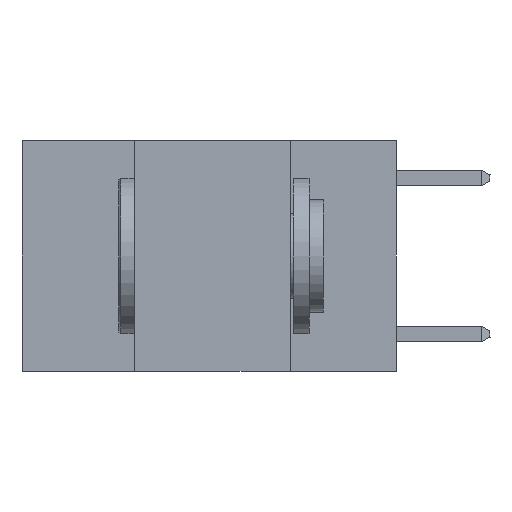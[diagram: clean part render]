
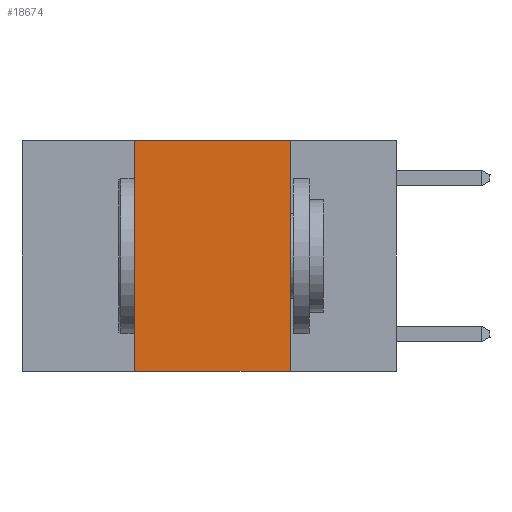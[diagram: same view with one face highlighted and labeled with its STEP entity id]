
A CAD part, left-side view. The second image highlights one B-rep face of the part: STEP entity #18674.
In plain terms, the highlighted planar face has unit normal (-1, 0, 0).
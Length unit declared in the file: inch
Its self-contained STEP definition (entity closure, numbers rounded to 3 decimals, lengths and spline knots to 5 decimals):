
#425 = LINE ( 'NONE', #23617, #4782 ) ;
#773 = VERTEX_POINT ( 'NONE', #7736 ) ;
#1393 = DIRECTION ( 'NONE',  ( 0., 0., -1. ) ) ;
#2004 = CARTESIAN_POINT ( 'NONE',  ( 0., 0.42, -0.37 ) ) ;
#2685 = VERTEX_POINT ( 'NONE', #2004 ) ;
#3588 = ORIENTED_EDGE ( 'NONE', *, *, #9557, .F. ) ;
#3977 = DIRECTION ( 'NONE',  ( 0., -1., 0. ) ) ;
#4782 = VECTOR ( 'NONE', #3977, 39.37008 ) ;
#5192 = DIRECTION ( 'NONE',  ( 1., 0., 0. ) ) ;
#5503 = VECTOR ( 'NONE', #1393, 39.37008 ) ;
#6861 = ORIENTED_EDGE ( 'NONE', *, *, #20769, .T. ) ;
#7736 = CARTESIAN_POINT ( 'NONE',  ( 0., 0.42, 0. ) ) ;
#7947 = VERTEX_POINT ( 'NONE', #11782 ) ;
#9023 = FACE_OUTER_BOUND ( 'NONE', #11222, .T. ) ;
#9557 = EDGE_CURVE ( 'NONE', #2685, #773, #24298, .T. ) ;
#10897 = LINE ( 'NONE', #11272, #5503 ) ;
#11222 = EDGE_LOOP ( 'NONE', ( #15689, #21444, #3588, #6861 ) ) ;
#11272 = CARTESIAN_POINT ( 'NONE',  ( 0., 0.17, 0. ) ) ;
#11639 = VECTOR ( 'NONE', #20247, 39.37008 ) ;
#11782 = CARTESIAN_POINT ( 'NONE',  ( 0., 0.17, -0.37 ) ) ;
#12774 = DIRECTION ( 'NONE',  ( 0., 0., 1. ) ) ;
#12934 = DIRECTION ( 'NONE',  ( 0., 0., -1. ) ) ;
#14403 = AXIS2_PLACEMENT_3D ( 'NONE', #14821, #5192, #12934 ) ;
#14821 = CARTESIAN_POINT ( 'NONE',  ( 0., 0.6, 0. ) ) ;
#15689 = ORIENTED_EDGE ( 'NONE', *, *, #18568, .F. ) ;
#16261 = CARTESIAN_POINT ( 'NONE',  ( 0., 0.17, 0. ) ) ;
#16722 = PLANE ( 'NONE',  #14403 ) ;
#18568 = EDGE_CURVE ( 'NONE', #24573, #7947, #10897, .T. ) ;
#18674 = ADVANCED_FACE ( 'NONE', ( #9023 ), #16722, .F. ) ;
#18940 = VECTOR ( 'NONE', #12774, 39.37008 ) ;
#20032 = EDGE_CURVE ( 'NONE', #773, #24573, #22052, .T. ) ;
#20247 = DIRECTION ( 'NONE',  ( 0., -1., 0. ) ) ;
#20769 = EDGE_CURVE ( 'NONE', #2685, #7947, #425, .T. ) ;
#21444 = ORIENTED_EDGE ( 'NONE', *, *, #20032, .F. ) ;
#22052 = LINE ( 'NONE', #23953, #11639 ) ;
#22905 = CARTESIAN_POINT ( 'NONE',  ( 0., 0.42, 0. ) ) ;
#23617 = CARTESIAN_POINT ( 'NONE',  ( 0., 0.6, -0.37 ) ) ;
#23953 = CARTESIAN_POINT ( 'NONE',  ( 0., 0.6, 0. ) ) ;
#24298 = LINE ( 'NONE', #22905, #18940 ) ;
#24573 = VERTEX_POINT ( 'NONE', #16261 ) ;
